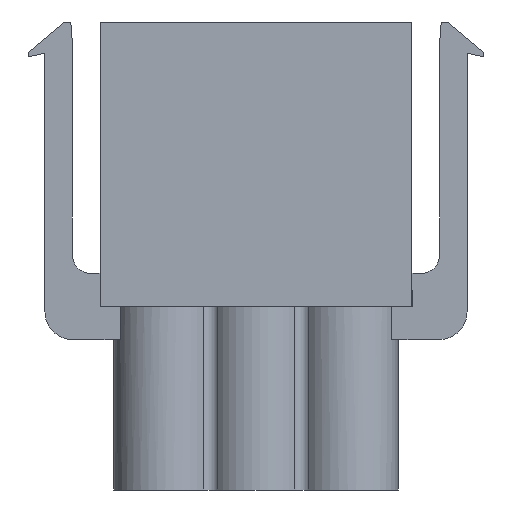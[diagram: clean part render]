
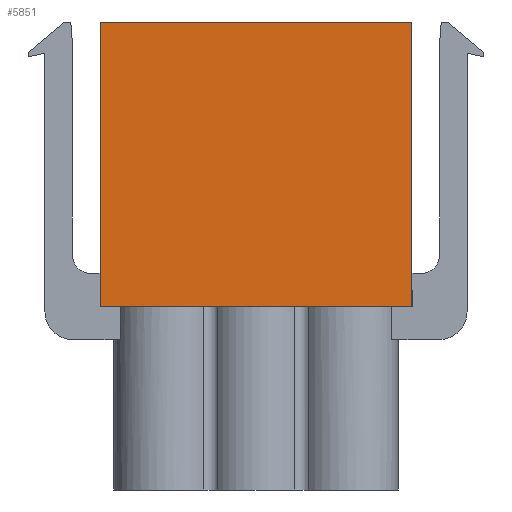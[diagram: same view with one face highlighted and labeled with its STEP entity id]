
A CAD part, front view. The second image highlights one B-rep face of the part: STEP entity #5851.
In plain terms, the highlighted planar face has unit normal (0, -1, 0).
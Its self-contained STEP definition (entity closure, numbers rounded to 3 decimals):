
#71 = CARTESIAN_POINT ( 'NONE',  ( 8.5, -4.05, -15.5 ) ) ;
#494 = CARTESIAN_POINT ( 'NONE',  ( 8.5, -4.05, 0. ) ) ;
#590 = CARTESIAN_POINT ( 'NONE',  ( -8.5, -4.05, -15.5 ) ) ;
#976 = EDGE_CURVE ( 'NONE', #4191, #5252, #2162, .T. ) ;
#1261 = EDGE_CURVE ( 'NONE', #4191, #6437, #8821, .T. ) ;
#1497 = CARTESIAN_POINT ( 'NONE',  ( -8.5, -4.05, -15.5 ) ) ;
#1663 = ORIENTED_EDGE ( 'NONE', *, *, #6603, .T. ) ;
#1788 = DIRECTION ( 'NONE',  ( 0., -1., 0. ) ) ;
#2054 = LINE ( 'NONE', #4074, #2102 ) ;
#2102 = VECTOR ( 'NONE', #5740, 1000. ) ;
#2162 = LINE ( 'NONE', #590, #5751 ) ;
#2335 = DIRECTION ( 'NONE',  ( 0., 0., -1. ) ) ;
#2728 = VERTEX_POINT ( 'NONE', #494 ) ;
#2927 = CARTESIAN_POINT ( 'NONE',  ( -8.5, -4.05, -15.5 ) ) ;
#3008 = EDGE_CURVE ( 'NONE', #6437, #2728, #2054, .T. ) ;
#3160 = ORIENTED_EDGE ( 'NONE', *, *, #3008, .F. ) ;
#3390 = DIRECTION ( 'NONE',  ( 0., 0., 1. ) ) ;
#3681 = DIRECTION ( 'NONE',  ( 1., 0., 0. ) ) ;
#3757 = FACE_OUTER_BOUND ( 'NONE', #9284, .T. ) ;
#3846 = ORIENTED_EDGE ( 'NONE', *, *, #1261, .F. ) ;
#3942 = VECTOR ( 'NONE', #3390, 1000. ) ;
#4036 = CARTESIAN_POINT ( 'NONE',  ( -8.5, -4.05, 0. ) ) ;
#4074 = CARTESIAN_POINT ( 'NONE',  ( -8.5, -4.05, 0. ) ) ;
#4191 = VERTEX_POINT ( 'NONE', #1497 ) ;
#4388 = CARTESIAN_POINT ( 'NONE',  ( -8.5, -4.05, -15.5 ) ) ;
#4603 = LINE ( 'NONE', #8678, #8842 ) ;
#5252 = VERTEX_POINT ( 'NONE', #71 ) ;
#5740 = DIRECTION ( 'NONE',  ( 1., 0., 0. ) ) ;
#5751 = VECTOR ( 'NONE', #3681, 1000. ) ;
#5851 = ADVANCED_FACE ( 'NONE', ( #3757 ), #8962, .T. ) ;
#6389 = DIRECTION ( 'NONE',  ( 0., 0., 1. ) ) ;
#6437 = VERTEX_POINT ( 'NONE', #4036 ) ;
#6524 = ORIENTED_EDGE ( 'NONE', *, *, #976, .T. ) ;
#6603 = EDGE_CURVE ( 'NONE', #5252, #2728, #4603, .T. ) ;
#7920 = AXIS2_PLACEMENT_3D ( 'NONE', #2927, #1788, #2335 ) ;
#8678 = CARTESIAN_POINT ( 'NONE',  ( 8.5, -4.05, -15.5 ) ) ;
#8821 = LINE ( 'NONE', #4388, #3942 ) ;
#8842 = VECTOR ( 'NONE', #6389, 1000. ) ;
#8962 = PLANE ( 'NONE',  #7920 ) ;
#9284 = EDGE_LOOP ( 'NONE', ( #3160, #3846, #6524, #1663 ) ) ;
